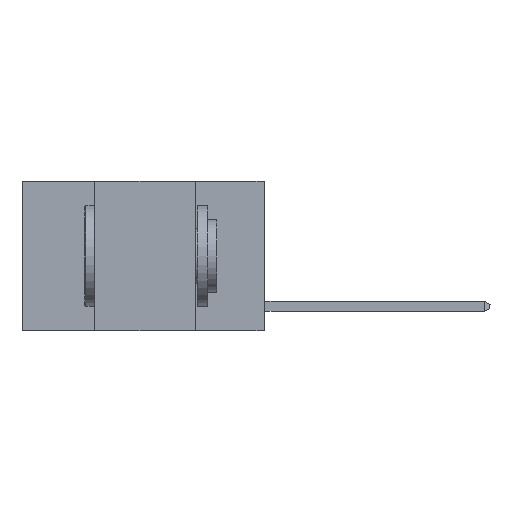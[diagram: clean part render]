
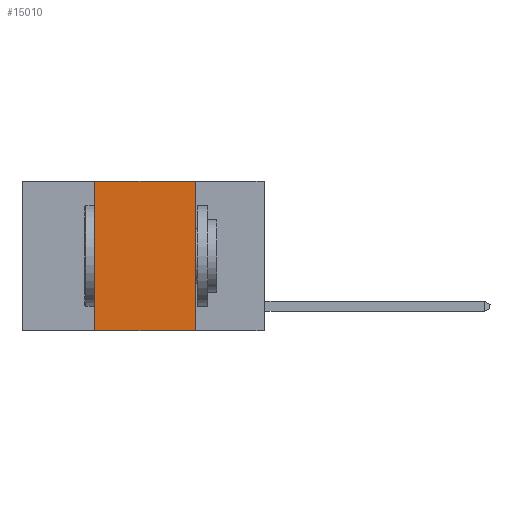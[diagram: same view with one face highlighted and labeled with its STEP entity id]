
A CAD part, left-side view. The second image highlights one B-rep face of the part: STEP entity #15010.
In plain terms, the highlighted planar face has unit normal (-1, 0, 0).
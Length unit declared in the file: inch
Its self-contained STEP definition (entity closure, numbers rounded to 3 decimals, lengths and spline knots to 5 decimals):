
#523 = EDGE_LOOP ( 'NONE', ( #8884, #5472, #22777, #14580 ) ) ;
#3451 = CARTESIAN_POINT ( 'NONE',  ( 0., 0.6, -0.37 ) ) ;
#3832 = LINE ( 'NONE', #22150, #4505 ) ;
#4505 = VECTOR ( 'NONE', #6123, 39.37008 ) ;
#4824 = EDGE_CURVE ( 'NONE', #24879, #12405, #10676, .T. ) ;
#5472 = ORIENTED_EDGE ( 'NONE', *, *, #17214, .F. ) ;
#6123 = DIRECTION ( 'NONE',  ( 0., -1., 0. ) ) ;
#7175 = DIRECTION ( 'NONE',  ( 0., 0., -1. ) ) ;
#7627 = DIRECTION ( 'NONE',  ( 0., 0., 1. ) ) ;
#8386 = DIRECTION ( 'NONE',  ( 0., 0., -1. ) ) ;
#8884 = ORIENTED_EDGE ( 'NONE', *, *, #4824, .F. ) ;
#10168 = CARTESIAN_POINT ( 'NONE',  ( 0., 0.42, 0. ) ) ;
#10676 = LINE ( 'NONE', #23028, #24166 ) ;
#11727 = LINE ( 'NONE', #3451, #18850 ) ;
#12405 = VERTEX_POINT ( 'NONE', #22641 ) ;
#14580 = ORIENTED_EDGE ( 'NONE', *, *, #26548, .T. ) ;
#15010 = ADVANCED_FACE ( 'NONE', ( #19907 ), #15594, .F. ) ;
#15594 = PLANE ( 'NONE',  #26110 ) ;
#16166 = LINE ( 'NONE', #17935, #17893 ) ;
#17214 = EDGE_CURVE ( 'NONE', #21846, #24879, #3832, .T. ) ;
#17733 = CARTESIAN_POINT ( 'NONE',  ( 0., 0.42, -0.37 ) ) ;
#17893 = VECTOR ( 'NONE', #7627, 39.37008 ) ;
#17935 = CARTESIAN_POINT ( 'NONE',  ( 0., 0.42, 0. ) ) ;
#18662 = CARTESIAN_POINT ( 'NONE',  ( 0., 0.17, 0. ) ) ;
#18850 = VECTOR ( 'NONE', #24340, 39.37008 ) ;
#19907 = FACE_OUTER_BOUND ( 'NONE', #523, .T. ) ;
#21846 = VERTEX_POINT ( 'NONE', #10168 ) ;
#22150 = CARTESIAN_POINT ( 'NONE',  ( 0., 0.6, 0. ) ) ;
#22502 = EDGE_CURVE ( 'NONE', #24656, #21846, #16166, .T. ) ;
#22641 = CARTESIAN_POINT ( 'NONE',  ( 0., 0.17, -0.37 ) ) ;
#22777 = ORIENTED_EDGE ( 'NONE', *, *, #22502, .F. ) ;
#23028 = CARTESIAN_POINT ( 'NONE',  ( 0., 0.17, 0. ) ) ;
#24166 = VECTOR ( 'NONE', #8386, 39.37008 ) ;
#24340 = DIRECTION ( 'NONE',  ( 0., -1., 0. ) ) ;
#24656 = VERTEX_POINT ( 'NONE', #17733 ) ;
#24879 = VERTEX_POINT ( 'NONE', #18662 ) ;
#25766 = DIRECTION ( 'NONE',  ( 1., 0., 0. ) ) ;
#26110 = AXIS2_PLACEMENT_3D ( 'NONE', #26165, #25766, #7175 ) ;
#26165 = CARTESIAN_POINT ( 'NONE',  ( 0., 0.6, 0. ) ) ;
#26548 = EDGE_CURVE ( 'NONE', #24656, #12405, #11727, .T. ) ;
